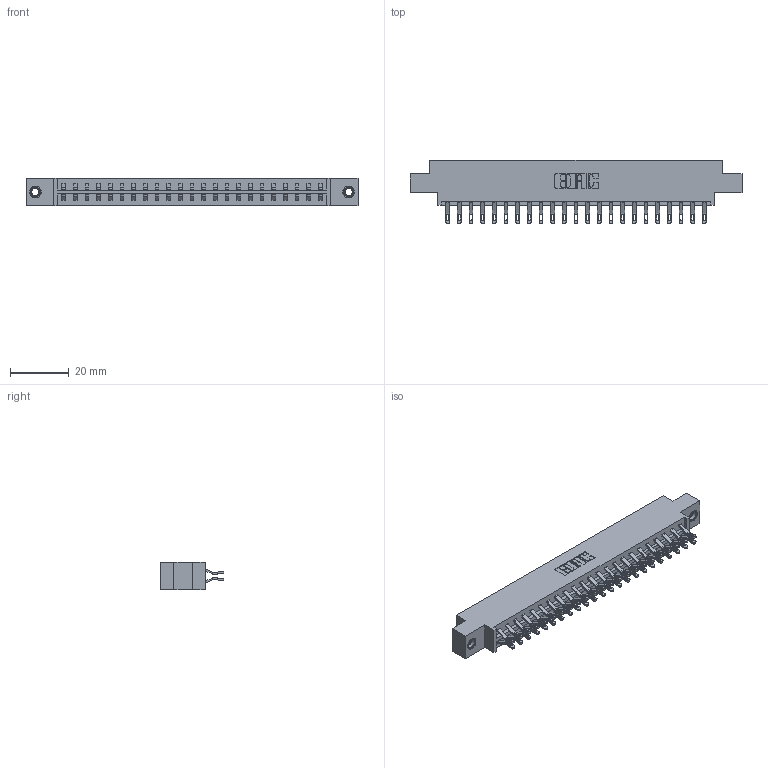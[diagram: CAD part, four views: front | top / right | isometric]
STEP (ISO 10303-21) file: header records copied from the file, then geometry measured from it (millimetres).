
FILE_DESCRIPTION (( 'STEP AP203' ), '1' );
FILE_NAME ('833-046-555-807.STEP', '2020-06-04T14:48:33', ( '' ), ( '' ), 'SwSTEP 2.0', 'SolidWorks 2020', '' );
FILE_SCHEMA (( 'CONFIG_CONTROL_DESIGN' ));
Length unit declared in the file: inch
Products named in the file (4): 833 Part_Offset - .156 Dia - TI; 833-046-555-807; 345-292-001_555 Tail; 345-250-001_345-250-005-103
Assembly tree (49 placements, depth 2):
  833-046-555-807
    833 Part_Offset - .156 Dia - TI
    345-292-001_555 Tail  x46
    345-250-001_345-250-005-103  x2
Bounding box: 112.67 x 21.47 x 9.4 mm (x, y, z)
Volume: 11217.8 mm3; surface area: 13812.1 mm2
Topology: 49 solids, 49 shells, 2846 faces, 8877 edges, 5910 vertices
Faces by surface type: plane 1670, cylinder 1160, cone 12, torus 4
Entity records: 18898 total; most frequent: CARTESIAN_POINT 3175, ORIENTED_EDGE 3074, DIRECTION 2747, EDGE_CURVE 1537, VECTOR 1369, LINE 1369, VERTEX_POINT 1020, AXIS2_PLACEMENT_3D 689
